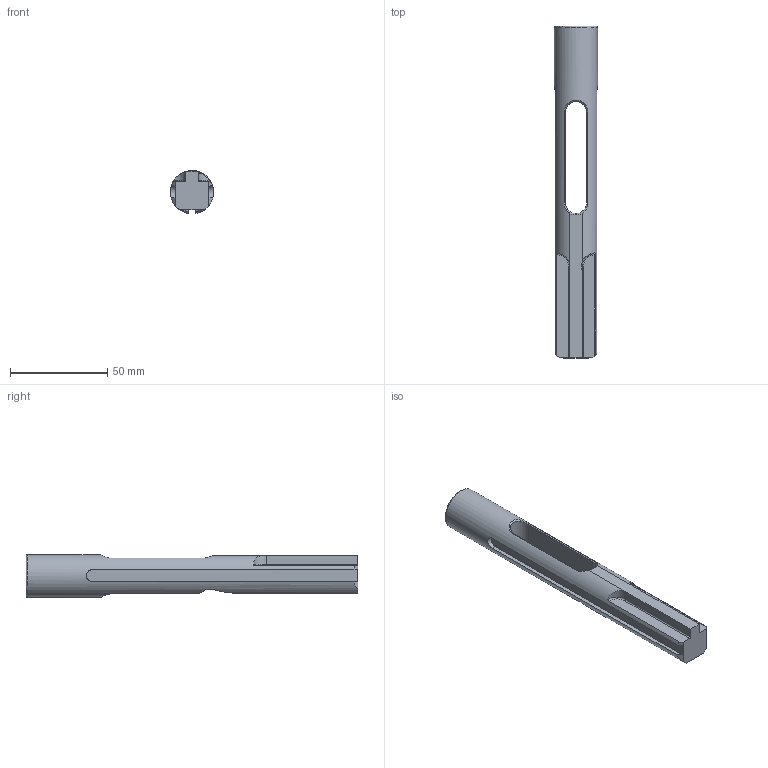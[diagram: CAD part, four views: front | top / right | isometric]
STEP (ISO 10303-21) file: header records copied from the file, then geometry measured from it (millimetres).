
FILE_DESCRIPTION(/* description */ ('','CAx-IF Rec.Pracs.---Representation and Presentation of Product Manufacturing Information (PMI)---4.0---2014-10-13'),/* implementation_level */ '2;1');
FILE_NAME(/* name */ 'Bolt Test v6.step',/* time_stamp */ '2025-01-30T00:28:07-07:00',/* author */ (''),/* organization */ (''),/* preprocessor_version */ 'ST-DEVELOPER v20',/* originating_system */ 'Autodesk Translation Framework v13.20.0.188',/* authorisation */ '');
FILE_SCHEMA (('AP242_MANAGED_MODEL_BASED_3D_ENGINEERING_MIM_LF { 1 0 10303 442 1 1 4 }'));
Length unit declared in the file: inch
Products named in the file (1): Bolt Test
Bounding box: 22.22 x 170.81 x 22.04 mm (x, y, z)
Volume: 44718 mm3; surface area: 15142.2 mm2
Topology: 1 solids, 1 shells, 48 faces, 136 edges, 88 vertices
Faces by surface type: plane 25, cylinder 10, bspline 8, torus 4, cone 1
Entity records: 2128 total; most frequent: CARTESIAN_POINT 923, ORIENTED_EDGE 272, DIRECTION 205, EDGE_CURVE 136, VERTEX_POINT 88, LINE 71, VECTOR 71, AXIS2_PLACEMENT_3D 67
